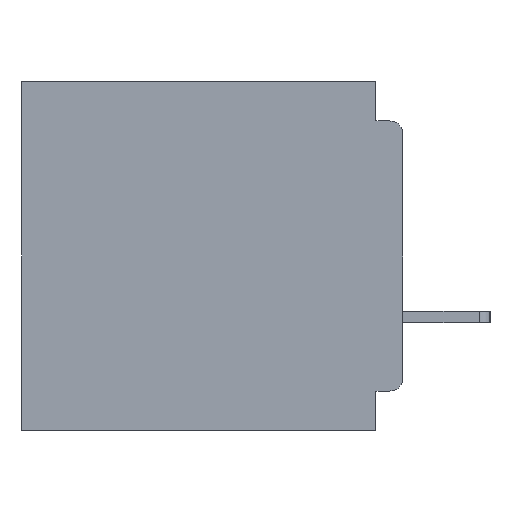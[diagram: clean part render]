
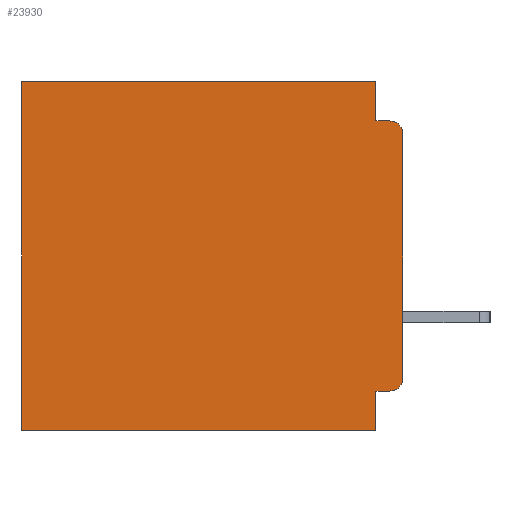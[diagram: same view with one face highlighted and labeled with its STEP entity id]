
A CAD part, left-side view. The second image highlights one B-rep face of the part: STEP entity #23930.
In plain terms, the highlighted planar face has unit normal (-1, 0, 0).
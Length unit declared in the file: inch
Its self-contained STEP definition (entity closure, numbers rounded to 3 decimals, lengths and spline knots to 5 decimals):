
#357 = CARTESIAN_POINT ( 'NONE',  ( 0.3, 0.437, 0. ) ) ;
#638 = DIRECTION ( 'NONE',  ( 1., 0., 0. ) ) ;
#1339 = LINE ( 'NONE', #34911, #26278 ) ;
#3571 = DIRECTION ( 'NONE',  ( 0., 0., -1. ) ) ;
#4237 = CARTESIAN_POINT ( 'NONE',  ( 0.3, 0., -0.34 ) ) ;
#4546 = AXIS2_PLACEMENT_3D ( 'NONE', #5832, #40476, #10893 ) ;
#4747 = EDGE_CURVE ( 'NONE', #44632, #8125, #37804, .T. ) ;
#4820 = AXIS2_PLACEMENT_3D ( 'NONE', #62510, #33278, #3571 ) ;
#5531 = DIRECTION ( 'NONE',  ( 0., 0., -1. ) ) ;
#5832 = CARTESIAN_POINT ( 'NONE',  ( 0.3, 0.015, -0.06 ) ) ;
#5957 = EDGE_CURVE ( 'NONE', #27940, #16214, #59101, .T. ) ;
#7485 = EDGE_CURVE ( 'NONE', #32350, #44632, #30283, .T. ) ;
#8125 = VERTEX_POINT ( 'NONE', #48612 ) ;
#8757 = ORIENTED_EDGE ( 'NONE', *, *, #21214, .F. ) ;
#9860 = CIRCLE ( 'NONE', #4820, 0.015 ) ;
#10714 = CARTESIAN_POINT ( 'NONE',  ( 0.3, 0., -0.4 ) ) ;
#10893 = DIRECTION ( 'NONE',  ( 0., 0., -1. ) ) ;
#10974 = LINE ( 'NONE', #40195, #35732 ) ;
#11064 = VECTOR ( 'NONE', #59420, 39.37008 ) ;
#11513 = VECTOR ( 'NONE', #26886, 39.37008 ) ;
#12823 = ORIENTED_EDGE ( 'NONE', *, *, #19799, .F. ) ;
#15734 = PLANE ( 'NONE',  #40247 ) ;
#16214 = VERTEX_POINT ( 'NONE', #50551 ) ;
#17229 = CARTESIAN_POINT ( 'NONE',  ( 0.3, 0.031, 0. ) ) ;
#18443 = DIRECTION ( 'NONE',  ( 0., 1., 0. ) ) ;
#18734 = CARTESIAN_POINT ( 'NONE',  ( 0.3, 0., 0. ) ) ;
#19799 = EDGE_CURVE ( 'NONE', #32350, #27940, #10974, .T. ) ;
#21214 = EDGE_CURVE ( 'NONE', #35566, #35038, #1339, .T. ) ;
#21519 = LINE ( 'NONE', #57186, #46145 ) ;
#21882 = ORIENTED_EDGE ( 'NONE', *, *, #24489, .T. ) ;
#22685 = ORIENTED_EDGE ( 'NONE', *, *, #41334, .T. ) ;
#23154 = VERTEX_POINT ( 'NONE', #4237 ) ;
#23164 = DIRECTION ( 'NONE',  ( 0., 1., 0. ) ) ;
#23930 = ADVANCED_FACE ( 'NONE', ( #46648 ), #15734, .F. ) ;
#24277 = LINE ( 'NONE', #44814, #11064 ) ;
#24489 = EDGE_CURVE ( 'NONE', #37294, #16214, #29738, .T. ) ;
#25611 = ORIENTED_EDGE ( 'NONE', *, *, #4747, .T. ) ;
#26278 = VECTOR ( 'NONE', #29990, 39.37008 ) ;
#26382 = CARTESIAN_POINT ( 'NONE',  ( 0.3, 0.437, -0.4 ) ) ;
#26886 = DIRECTION ( 'NONE',  ( 0., 0., -1. ) ) ;
#27516 = DIRECTION ( 'NONE',  ( 0., 0., -1. ) ) ;
#27575 = VECTOR ( 'NONE', #27516, 39.37008 ) ;
#27928 = ORIENTED_EDGE ( 'NONE', *, *, #29484, .F. ) ;
#27940 = VERTEX_POINT ( 'NONE', #45057 ) ;
#29484 = EDGE_CURVE ( 'NONE', #35038, #44330, #39124, .T. ) ;
#29738 = CIRCLE ( 'NONE', #4546, 0.015 ) ;
#29990 = DIRECTION ( 'NONE',  ( 0., 1., 0. ) ) ;
#30283 = LINE ( 'NONE', #18734, #41773 ) ;
#30490 = ORIENTED_EDGE ( 'NONE', *, *, #63148, .F. ) ;
#32350 = VERTEX_POINT ( 'NONE', #17229 ) ;
#33278 = DIRECTION ( 'NONE',  ( -1., 0., 0. ) ) ;
#34911 = CARTESIAN_POINT ( 'NONE',  ( 0.3, 0., -0.355 ) ) ;
#35038 = VERTEX_POINT ( 'NONE', #36673 ) ;
#35566 = VERTEX_POINT ( 'NONE', #45434 ) ;
#35732 = VECTOR ( 'NONE', #5531, 39.37008 ) ;
#36229 = VECTOR ( 'NONE', #54735, 39.37008 ) ;
#36673 = CARTESIAN_POINT ( 'NONE',  ( 0.3, 0.031, -0.355 ) ) ;
#37294 = VERTEX_POINT ( 'NONE', #58934 ) ;
#37729 = EDGE_LOOP ( 'NONE', ( #47664, #21882, #44926, #12823, #39544, #25611, #30490, #27928, #8757, #22685 ) ) ;
#37804 = LINE ( 'NONE', #26382, #11513 ) ;
#37935 = CARTESIAN_POINT ( 'NONE',  ( 0.3, 0.031, -0.4 ) ) ;
#38472 = EDGE_CURVE ( 'NONE', #37294, #23154, #24277, .T. ) ;
#39124 = LINE ( 'NONE', #56833, #27575 ) ;
#39544 = ORIENTED_EDGE ( 'NONE', *, *, #7485, .T. ) ;
#40195 = CARTESIAN_POINT ( 'NONE',  ( 0.3, 0.031, 0. ) ) ;
#40247 = AXIS2_PLACEMENT_3D ( 'NONE', #10714, #638, #50187 ) ;
#40476 = DIRECTION ( 'NONE',  ( -1., 0., 0. ) ) ;
#41334 = EDGE_CURVE ( 'NONE', #35566, #23154, #9860, .T. ) ;
#41773 = VECTOR ( 'NONE', #18443, 39.37008 ) ;
#44330 = VERTEX_POINT ( 'NONE', #37935 ) ;
#44632 = VERTEX_POINT ( 'NONE', #357 ) ;
#44814 = CARTESIAN_POINT ( 'NONE',  ( 0.3, 0., -0.4 ) ) ;
#44926 = ORIENTED_EDGE ( 'NONE', *, *, #5957, .F. ) ;
#45057 = CARTESIAN_POINT ( 'NONE',  ( 0.3, 0.031, -0.045 ) ) ;
#45434 = CARTESIAN_POINT ( 'NONE',  ( 0.3, 0.015, -0.355 ) ) ;
#46145 = VECTOR ( 'NONE', #23164, 39.37008 ) ;
#46648 = FACE_OUTER_BOUND ( 'NONE', #37729, .T. ) ;
#47664 = ORIENTED_EDGE ( 'NONE', *, *, #38472, .F. ) ;
#48612 = CARTESIAN_POINT ( 'NONE',  ( 0.3, 0.437, -0.4 ) ) ;
#50187 = DIRECTION ( 'NONE',  ( 0., 0., -1. ) ) ;
#50551 = CARTESIAN_POINT ( 'NONE',  ( 0.3, 0.015, -0.045 ) ) ;
#54678 = CARTESIAN_POINT ( 'NONE',  ( 0.3, 0., -0.045 ) ) ;
#54735 = DIRECTION ( 'NONE',  ( 0., -1., 0. ) ) ;
#56833 = CARTESIAN_POINT ( 'NONE',  ( 0.3, 0.031, -0.4 ) ) ;
#57186 = CARTESIAN_POINT ( 'NONE',  ( 0.3, 0., -0.4 ) ) ;
#58934 = CARTESIAN_POINT ( 'NONE',  ( 0.3, 0., -0.06 ) ) ;
#59101 = LINE ( 'NONE', #54678, #36229 ) ;
#59420 = DIRECTION ( 'NONE',  ( 0., 0., -1. ) ) ;
#62510 = CARTESIAN_POINT ( 'NONE',  ( 0.3, 0.015, -0.34 ) ) ;
#63148 = EDGE_CURVE ( 'NONE', #44330, #8125, #21519, .T. ) ;
